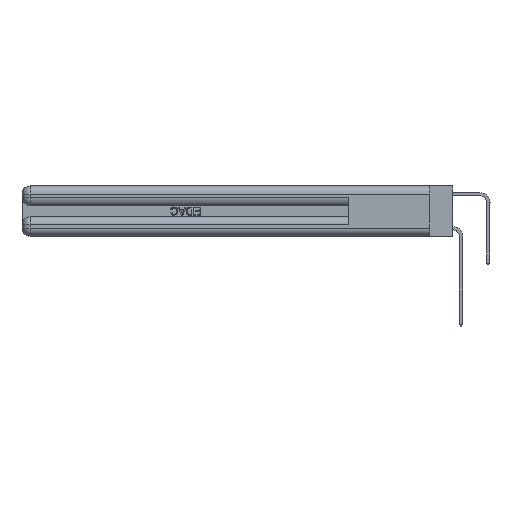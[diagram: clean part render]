
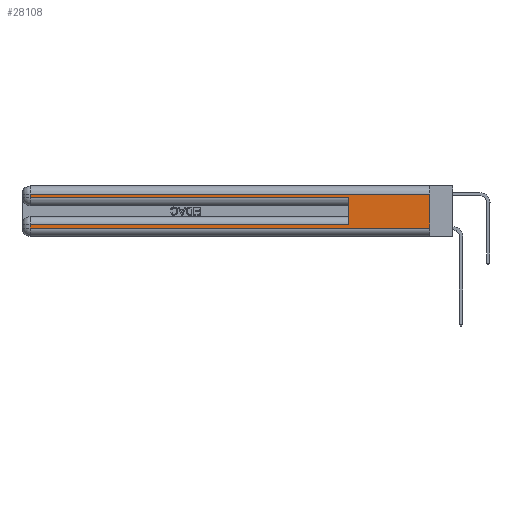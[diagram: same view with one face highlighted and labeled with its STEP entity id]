
A CAD part, left-side view. The second image highlights one B-rep face of the part: STEP entity #28108.
In plain terms, the highlighted planar face has unit normal (-1, 0, 0).
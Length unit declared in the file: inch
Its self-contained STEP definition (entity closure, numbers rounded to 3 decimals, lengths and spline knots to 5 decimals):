
#391 = DIRECTION ( 'NONE',  ( 1., 0., 0. ) ) ;
#693 = EDGE_CURVE ( 'NONE', #21747, #13009, #15836, .T. ) ;
#987 = FACE_OUTER_BOUND ( 'NONE', #26418, .T. ) ;
#1639 = DIRECTION ( 'NONE',  ( 0., 1., 0. ) ) ;
#1680 = CARTESIAN_POINT ( 'NONE',  ( 0., 2.94, 0.085 ) ) ;
#1761 = CARTESIAN_POINT ( 'NONE',  ( 0., 0., 0.31 ) ) ;
#2457 = VERTEX_POINT ( 'NONE', #7533 ) ;
#3142 = CARTESIAN_POINT ( 'NONE',  ( 0., 0., 0.06 ) ) ;
#3971 = VERTEX_POINT ( 'NONE', #3142 ) ;
#4746 = CARTESIAN_POINT ( 'NONE',  ( 0., 2.94, 0.37 ) ) ;
#4854 = ORIENTED_EDGE ( 'NONE', *, *, #32554, .T. ) ;
#5519 = EDGE_CURVE ( 'NONE', #35161, #8800, #28810, .T. ) ;
#6100 = CARTESIAN_POINT ( 'NONE',  ( 0., 2.94, 0.06 ) ) ;
#7001 = LINE ( 'NONE', #11929, #11775 ) ;
#7533 = CARTESIAN_POINT ( 'NONE',  ( 0., 0.6, 0.285 ) ) ;
#7604 = LINE ( 'NONE', #28073, #13232 ) ;
#7751 = CARTESIAN_POINT ( 'NONE',  ( 0., 0., 0.37 ) ) ;
#8594 = ORIENTED_EDGE ( 'NONE', *, *, #12521, .F. ) ;
#8596 = LINE ( 'NONE', #23209, #26433 ) ;
#8800 = VERTEX_POINT ( 'NONE', #1680 ) ;
#9210 = EDGE_CURVE ( 'NONE', #32277, #21747, #19754, .T. ) ;
#9542 = DIRECTION ( 'NONE',  ( 0., -1., 0. ) ) ;
#10537 = EDGE_CURVE ( 'NONE', #30689, #3971, #32720, .T. ) ;
#11098 = CARTESIAN_POINT ( 'NONE',  ( 0., 0., 0.085 ) ) ;
#11702 = VECTOR ( 'NONE', #34920, 39.37008 ) ;
#11775 = VECTOR ( 'NONE', #9542, 39.37008 ) ;
#11929 = CARTESIAN_POINT ( 'NONE',  ( 0., 0., 0.285 ) ) ;
#12521 = EDGE_CURVE ( 'NONE', #35161, #2457, #8596, .T. ) ;
#12714 = PLANE ( 'NONE',  #26796 ) ;
#13009 = VERTEX_POINT ( 'NONE', #13165 ) ;
#13108 = ORIENTED_EDGE ( 'NONE', *, *, #33304, .T. ) ;
#13165 = CARTESIAN_POINT ( 'NONE',  ( 0., 2.94, 0.285 ) ) ;
#13232 = VECTOR ( 'NONE', #25004, 39.37008 ) ;
#14906 = EDGE_CURVE ( 'NONE', #32277, #3971, #7604, .T. ) ;
#15836 = LINE ( 'NONE', #4746, #34552 ) ;
#17607 = DIRECTION ( 'NONE',  ( 0., -1., 0. ) ) ;
#17641 = DIRECTION ( 'NONE',  ( 0., 0., 1. ) ) ;
#19500 = DIRECTION ( 'NONE',  ( 0., 1., 0. ) ) ;
#19754 = LINE ( 'NONE', #1761, #33676 ) ;
#19833 = ORIENTED_EDGE ( 'NONE', *, *, #10537, .T. ) ;
#20919 = VECTOR ( 'NONE', #19500, 39.37008 ) ;
#20954 = ORIENTED_EDGE ( 'NONE', *, *, #14906, .F. ) ;
#21747 = VERTEX_POINT ( 'NONE', #35157 ) ;
#22132 = ORIENTED_EDGE ( 'NONE', *, *, #5519, .T. ) ;
#22236 = ORIENTED_EDGE ( 'NONE', *, *, #9210, .T. ) ;
#23209 = CARTESIAN_POINT ( 'NONE',  ( 0., 0.6, 0.145 ) ) ;
#23457 = CARTESIAN_POINT ( 'NONE',  ( 0., 2.94, 0.37 ) ) ;
#24626 = CARTESIAN_POINT ( 'NONE',  ( 0., 0.6, 0.085 ) ) ;
#25004 = DIRECTION ( 'NONE',  ( 0., 0., -1. ) ) ;
#26418 = EDGE_LOOP ( 'NONE', ( #20954, #22236, #28367, #4854, #8594, #22132, #13108, #19833 ) ) ;
#26433 = VECTOR ( 'NONE', #17641, 39.37008 ) ;
#26796 = AXIS2_PLACEMENT_3D ( 'NONE', #7751, #391, #27320 ) ;
#27143 = DIRECTION ( 'NONE',  ( 0., 0., -1. ) ) ;
#27320 = DIRECTION ( 'NONE',  ( 0., 0., -1. ) ) ;
#28073 = CARTESIAN_POINT ( 'NONE',  ( 0., 0., 0.37 ) ) ;
#28108 = ADVANCED_FACE ( 'NONE', ( #987 ), #12714, .F. ) ;
#28367 = ORIENTED_EDGE ( 'NONE', *, *, #693, .T. ) ;
#28810 = LINE ( 'NONE', #11098, #20919 ) ;
#29158 = LINE ( 'NONE', #23457, #11702 ) ;
#30523 = VECTOR ( 'NONE', #17607, 39.37008 ) ;
#30689 = VERTEX_POINT ( 'NONE', #6100 ) ;
#31506 = CARTESIAN_POINT ( 'NONE',  ( 0., 0., 0.06 ) ) ;
#32277 = VERTEX_POINT ( 'NONE', #35597 ) ;
#32554 = EDGE_CURVE ( 'NONE', #13009, #2457, #7001, .T. ) ;
#32720 = LINE ( 'NONE', #31506, #30523 ) ;
#33304 = EDGE_CURVE ( 'NONE', #8800, #30689, #29158, .T. ) ;
#33676 = VECTOR ( 'NONE', #1639, 39.37008 ) ;
#34552 = VECTOR ( 'NONE', #27143, 39.37008 ) ;
#34920 = DIRECTION ( 'NONE',  ( 0., 0., -1. ) ) ;
#35157 = CARTESIAN_POINT ( 'NONE',  ( 0., 2.94, 0.31 ) ) ;
#35161 = VERTEX_POINT ( 'NONE', #24626 ) ;
#35597 = CARTESIAN_POINT ( 'NONE',  ( 0., 0., 0.31 ) ) ;
